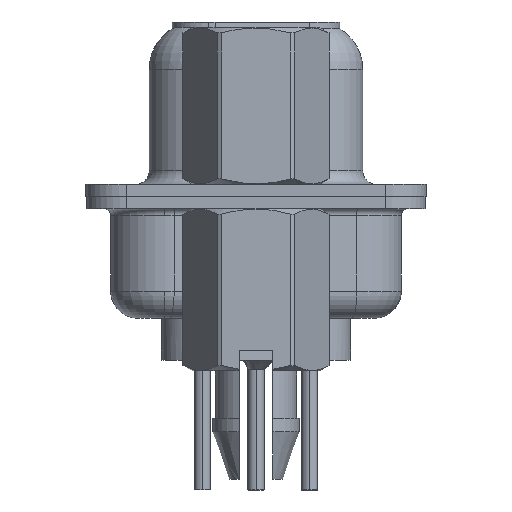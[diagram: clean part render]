
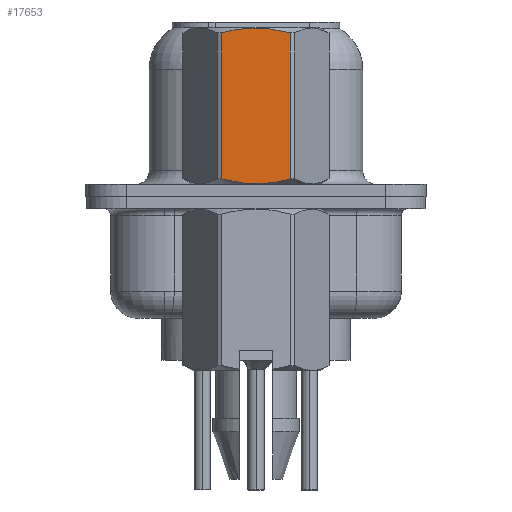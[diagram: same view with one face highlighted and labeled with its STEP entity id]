
A CAD part, left-side view. The second image highlights one B-rep face of the part: STEP entity #17653.
In plain terms, the highlighted planar face has unit normal (-1, 0, 0).
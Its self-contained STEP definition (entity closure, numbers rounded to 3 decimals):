
#435 = VERTEX_POINT ( 'NONE', #15488 ) ;
#1068 = VERTEX_POINT ( 'NONE', #27765 ) ;
#2255 = CARTESIAN_POINT ( 'NONE',  ( -2.381, 0.215, 0.468 ) ) ;
#3187 = LINE ( 'NONE', #16000, #30600 ) ;
#3910 = CARTESIAN_POINT ( 'NONE',  ( -2.381, -1.273, 6.048 ) ) ;
#4130 = FACE_OUTER_BOUND ( 'NONE', #26872, .T. ) ;
#4989 = CARTESIAN_POINT ( 'NONE',  ( -2.381, -0.432, 0.485 ) ) ;
#6146 = ORIENTED_EDGE ( 'NONE', *, *, #14038, .T. ) ;
#7678 = CARTESIAN_POINT ( 'NONE',  ( -2.381, -1.066, 0.596 ) ) ;
#9062 = CARTESIAN_POINT ( 'NONE',  ( -2.381, -1.066, 6.104 ) ) ;
#9294 = CARTESIAN_POINT ( 'NONE',  ( -2.381, -0.432, 6.215 ) ) ;
#10130 = ORIENTED_EDGE ( 'NONE', *, *, #10647, .T. ) ;
#10482 = EDGE_CURVE ( 'NONE', #27457, #1068, #20070, .T. ) ;
#10647 = EDGE_CURVE ( 'NONE', #435, #27457, #3187, .T. ) ;
#11995 = CARTESIAN_POINT ( 'NONE',  ( -2.381, 0.215, 6.232 ) ) ;
#12038 = PLANE ( 'NONE',  #22150 ) ;
#12279 = DIRECTION ( 'NONE',  ( -1., 0., 0. ) ) ;
#12917 = ORIENTED_EDGE ( 'NONE', *, *, #10482, .T. ) ;
#14038 = EDGE_CURVE ( 'NONE', #22485, #435, #16109, .T. ) ;
#14667 = CARTESIAN_POINT ( 'NONE',  ( -2.381, 0.853, 6.151 ) ) ;
#15488 = CARTESIAN_POINT ( 'NONE',  ( -2.381, 1.273, 6.048 ) ) ;
#15591 = CARTESIAN_POINT ( 'NONE',  ( -2.381, 1.273, 0.652 ) ) ;
#16000 = CARTESIAN_POINT ( 'NONE',  ( -2.381, 1.273, 3.792 ) ) ;
#16109 = B_SPLINE_CURVE_WITH_KNOTS ( 'NONE', 3,
 ( #3910, #9062, #25171, #9294, #27814, #11995, #30467, #14667, #33104, #17315 ),
 .UNSPECIFIED., .F., .F.,
 ( 4, 2, 2, 2, 4 ),
 ( 0.001, 0.002, 0.002, 0.003, 0.004 ),
 .UNSPECIFIED. ) ;
#17315 = CARTESIAN_POINT ( 'NONE',  ( -2.381, 1.273, 6.048 ) ) ;
#17653 = ADVANCED_FACE ( 'NONE', ( #4130 ), #12038, .T. ) ;
#18241 = EDGE_CURVE ( 'NONE', #1068, #22485, #28602, .T. ) ;
#18254 = CARTESIAN_POINT ( 'NONE',  ( -2.381, 0.428, 0.485 ) ) ;
#19934 = VECTOR ( 'NONE', #30252, 1000. ) ;
#20070 = B_SPLINE_CURVE_WITH_KNOTS ( 'NONE', 3,
 ( #15591, #31396, #34040, #18254, #2255, #20916, #4989, #23554, #7678, #26217 ),
 .UNSPECIFIED., .F., .F.,
 ( 4, 2, 2, 2, 4 ),
 ( 0.003, 0.003, 0.004, 0.004, 0.005 ),
 .UNSPECIFIED. ) ;
#20916 = CARTESIAN_POINT ( 'NONE',  ( -2.381, -0.215, 0.468 ) ) ;
#21084 = CARTESIAN_POINT ( 'NONE',  ( -2.381, -1.273, 6.048 ) ) ;
#22150 = AXIS2_PLACEMENT_3D ( 'NONE', #28096, #12279, #30755 ) ;
#22485 = VERTEX_POINT ( 'NONE', #21084 ) ;
#23547 = CARTESIAN_POINT ( 'NONE',  ( -2.381, 1.273, 0.652 ) ) ;
#23554 = CARTESIAN_POINT ( 'NONE',  ( -2.381, -0.858, 0.55 ) ) ;
#23833 = ORIENTED_EDGE ( 'NONE', *, *, #18241, .T. ) ;
#25171 = CARTESIAN_POINT ( 'NONE',  ( -2.381, -0.858, 6.15 ) ) ;
#26217 = CARTESIAN_POINT ( 'NONE',  ( -2.381, -1.273, 0.652 ) ) ;
#26500 = DIRECTION ( 'NONE',  ( 0., 0., -1. ) ) ;
#26872 = EDGE_LOOP ( 'NONE', ( #12917, #23833, #6146, #10130 ) ) ;
#27457 = VERTEX_POINT ( 'NONE', #23547 ) ;
#27765 = CARTESIAN_POINT ( 'NONE',  ( -2.381, -1.273, 0.652 ) ) ;
#27814 = CARTESIAN_POINT ( 'NONE',  ( -2.381, -0.215, 6.232 ) ) ;
#28096 = CARTESIAN_POINT ( 'NONE',  ( -2.381, 1.375, -3.75 ) ) ;
#28602 = LINE ( 'NONE', #33005, #19934 ) ;
#30252 = DIRECTION ( 'NONE',  ( 0., 0., 1. ) ) ;
#30467 = CARTESIAN_POINT ( 'NONE',  ( -2.381, 0.428, 6.215 ) ) ;
#30600 = VECTOR ( 'NONE', #26500, 1000. ) ;
#30755 = DIRECTION ( 'NONE',  ( 0., -1., 0. ) ) ;
#31396 = CARTESIAN_POINT ( 'NONE',  ( -2.381, 1.065, 0.596 ) ) ;
#33005 = CARTESIAN_POINT ( 'NONE',  ( -2.381, -1.273, 3.792 ) ) ;
#33104 = CARTESIAN_POINT ( 'NONE',  ( -2.381, 1.065, 6.104 ) ) ;
#34040 = CARTESIAN_POINT ( 'NONE',  ( -2.381, 0.853, 0.549 ) ) ;
